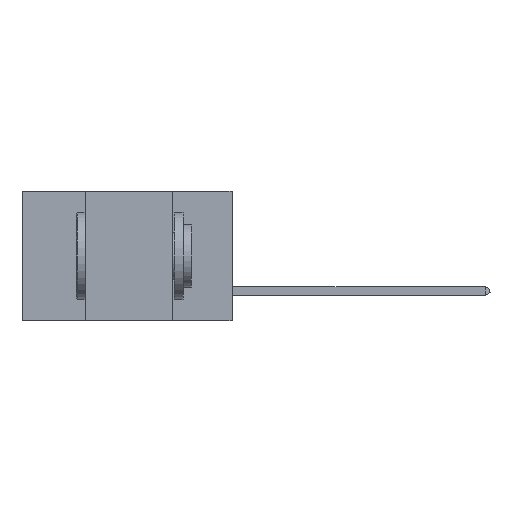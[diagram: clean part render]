
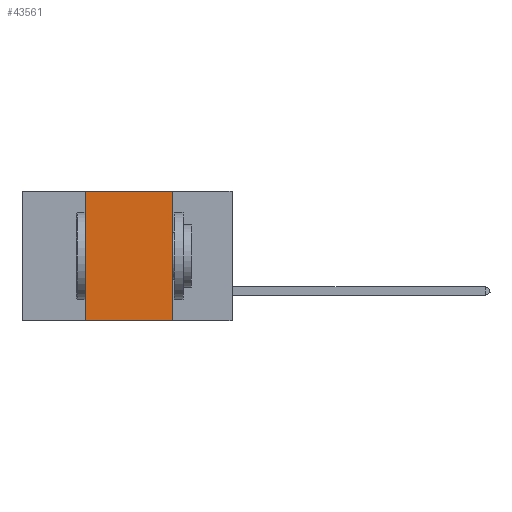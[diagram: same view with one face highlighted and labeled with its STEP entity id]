
A CAD part, left-side view. The second image highlights one B-rep face of the part: STEP entity #43561.
In plain terms, the highlighted planar face has unit normal (-1, 0, 0).
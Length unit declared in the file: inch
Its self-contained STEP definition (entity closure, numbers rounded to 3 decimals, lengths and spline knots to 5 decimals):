
#1732 = EDGE_LOOP ( 'NONE', ( #6387, #28330, #21238, #15073 ) ) ;
#1960 = LINE ( 'NONE', #18404, #23794 ) ;
#2041 = VECTOR ( 'NONE', #2927, 39.37008 ) ;
#2927 = DIRECTION ( 'NONE',  ( 0., -1., 0. ) ) ;
#2975 = CARTESIAN_POINT ( 'NONE',  ( 0., 0.17, 0. ) ) ;
#3919 = EDGE_CURVE ( 'NONE', #23855, #7236, #1960, .T. ) ;
#5083 = CARTESIAN_POINT ( 'NONE',  ( 0., 0.17, 0. ) ) ;
#5884 = EDGE_CURVE ( 'NONE', #7236, #44130, #32419, .T. ) ;
#6387 = ORIENTED_EDGE ( 'NONE', *, *, #25690, .F. ) ;
#7021 = DIRECTION ( 'NONE',  ( 0., 0., 1. ) ) ;
#7236 = VERTEX_POINT ( 'NONE', #48588 ) ;
#8119 = EDGE_CURVE ( 'NONE', #23855, #23547, #25679, .T. ) ;
#10868 = CARTESIAN_POINT ( 'NONE',  ( 0., 0.6, -0.37 ) ) ;
#11118 = DIRECTION ( 'NONE',  ( 1., 0., 0. ) ) ;
#12150 = LINE ( 'NONE', #5083, #35773 ) ;
#12359 = VECTOR ( 'NONE', #46672, 39.37008 ) ;
#12672 = DIRECTION ( 'NONE',  ( 0., 0., -1. ) ) ;
#15073 = ORIENTED_EDGE ( 'NONE', *, *, #8119, .T. ) ;
#18404 = CARTESIAN_POINT ( 'NONE',  ( 0., 0.42, 0. ) ) ;
#21238 = ORIENTED_EDGE ( 'NONE', *, *, #3919, .F. ) ;
#23547 = VERTEX_POINT ( 'NONE', #39337 ) ;
#23611 = CARTESIAN_POINT ( 'NONE',  ( 0., 0.6, 0. ) ) ;
#23794 = VECTOR ( 'NONE', #7021, 39.37008 ) ;
#23855 = VERTEX_POINT ( 'NONE', #33245 ) ;
#25679 = LINE ( 'NONE', #10868, #2041 ) ;
#25690 = EDGE_CURVE ( 'NONE', #44130, #23547, #12150, .T. ) ;
#25980 = DIRECTION ( 'NONE',  ( 0., 0., -1. ) ) ;
#28330 = ORIENTED_EDGE ( 'NONE', *, *, #5884, .F. ) ;
#32419 = LINE ( 'NONE', #23611, #12359 ) ;
#32572 = AXIS2_PLACEMENT_3D ( 'NONE', #37666, #11118, #25980 ) ;
#32689 = FACE_OUTER_BOUND ( 'NONE', #1732, .T. ) ;
#33245 = CARTESIAN_POINT ( 'NONE',  ( 0., 0.42, -0.37 ) ) ;
#35773 = VECTOR ( 'NONE', #12672, 39.37008 ) ;
#37666 = CARTESIAN_POINT ( 'NONE',  ( 0., 0.6, 0. ) ) ;
#39337 = CARTESIAN_POINT ( 'NONE',  ( 0., 0.17, -0.37 ) ) ;
#43561 = ADVANCED_FACE ( 'NONE', ( #32689 ), #48534, .F. ) ;
#44130 = VERTEX_POINT ( 'NONE', #2975 ) ;
#46672 = DIRECTION ( 'NONE',  ( 0., -1., 0. ) ) ;
#48534 = PLANE ( 'NONE',  #32572 ) ;
#48588 = CARTESIAN_POINT ( 'NONE',  ( 0., 0.42, 0. ) ) ;
